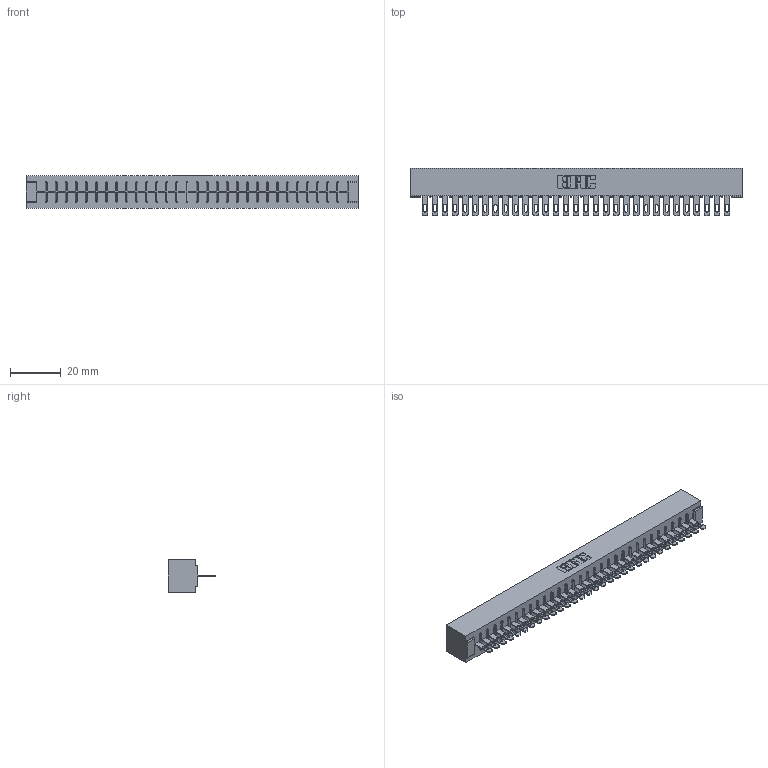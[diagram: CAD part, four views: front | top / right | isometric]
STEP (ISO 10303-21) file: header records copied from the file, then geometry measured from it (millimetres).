
FILE_DESCRIPTION (( 'STEP AP203' ), '1' );
FILE_NAME ('316-031-500-101.STEP', '2018-07-31T03:24:30', ( '' ), ( '' ), 'SwSTEP 2.0', 'SolidWorks 2016', '' );
FILE_SCHEMA (( 'CONFIG_CONTROL_DESIGN' ));
Length unit declared in the file: inch
Products named in the file (3): 306-290-001_100; 316-031-500-101; 306 Part_No Mounting
Assembly tree (32 placements, depth 2):
  316-031-500-101
    306 Part_No Mounting
    306-290-001_100  x31
Bounding box: 130.71 x 18.87 x 12.7 mm (x, y, z)
Volume: 15039.2 mm3; surface area: 15993.5 mm2
Topology: 32 solids, 32 shells, 2464 faces, 6957 edges, 4470 vertices
Faces by surface type: plane 1614, cylinder 726, sphere 124
Entity records: 30220 total; most frequent: CARTESIAN_POINT 5072, ORIENTED_EDGE 5026, DIRECTION 5003, EDGE_CURVE 2513, VECTOR 1961, LINE 1961, VERTEX_POINT 1590, AXIS2_PLACEMENT_3D 1521
